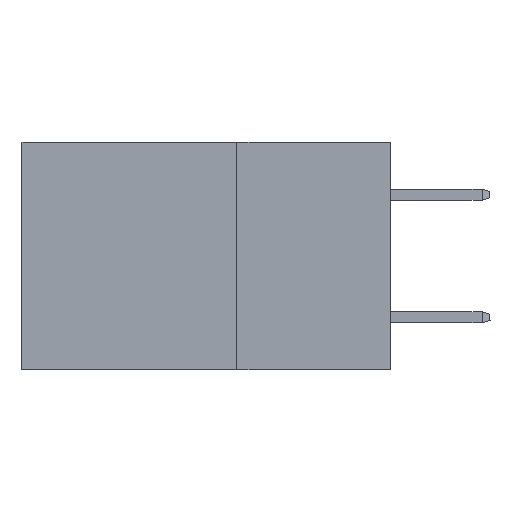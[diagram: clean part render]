
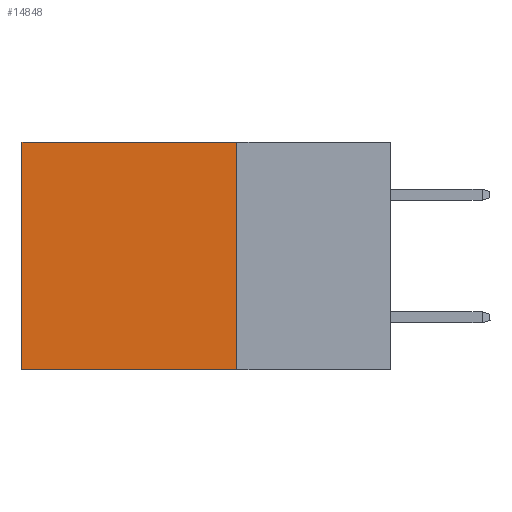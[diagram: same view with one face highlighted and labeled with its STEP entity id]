
A CAD part, left-side view. The second image highlights one B-rep face of the part: STEP entity #14848.
In plain terms, the highlighted planar face has unit normal (-1, 0, 0).
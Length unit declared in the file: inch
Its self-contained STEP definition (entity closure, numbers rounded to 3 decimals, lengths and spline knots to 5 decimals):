
#57 = EDGE_CURVE ( 'NONE', #25515, #14974, #1301, .T. ) ;
#1301 = LINE ( 'NONE', #20727, #3174 ) ;
#2214 = LINE ( 'NONE', #20636, #16234 ) ;
#3174 = VECTOR ( 'NONE', #24867, 39.37008 ) ;
#4526 = VECTOR ( 'NONE', #22218, 39.37008 ) ;
#6023 = CARTESIAN_POINT ( 'NONE',  ( 0.2875, 0.25, -0.37 ) ) ;
#7574 = EDGE_LOOP ( 'NONE', ( #11862, #17883, #24803, #11158 ) ) ;
#7950 = LINE ( 'NONE', #10287, #4526 ) ;
#8965 = PLANE ( 'NONE',  #15084 ) ;
#9404 = VECTOR ( 'NONE', #16774, 39.37008 ) ;
#10287 = CARTESIAN_POINT ( 'NONE',  ( 0.2875, 0.25, -0.37 ) ) ;
#10639 = DIRECTION ( 'NONE',  ( 0., 0., -1. ) ) ;
#11158 = ORIENTED_EDGE ( 'NONE', *, *, #15975, .T. ) ;
#11862 = ORIENTED_EDGE ( 'NONE', *, *, #57, .T. ) ;
#12198 = VERTEX_POINT ( 'NONE', #22595 ) ;
#14715 = LINE ( 'NONE', #20918, #9404 ) ;
#14848 = ADVANCED_FACE ( 'NONE', ( #20401 ), #8965, .F. ) ;
#14974 = VERTEX_POINT ( 'NONE', #17352 ) ;
#15084 = AXIS2_PLACEMENT_3D ( 'NONE', #18603, #22837, #10639 ) ;
#15472 = EDGE_CURVE ( 'NONE', #12198, #21016, #14715, .T. ) ;
#15975 = EDGE_CURVE ( 'NONE', #12198, #25515, #2214, .T. ) ;
#16234 = VECTOR ( 'NONE', #24873, 39.37008 ) ;
#16774 = DIRECTION ( 'NONE',  ( 0., 0., -1. ) ) ;
#17352 = CARTESIAN_POINT ( 'NONE',  ( 0.2875, 0.6, -0.37 ) ) ;
#17883 = ORIENTED_EDGE ( 'NONE', *, *, #23060, .F. ) ;
#18603 = CARTESIAN_POINT ( 'NONE',  ( 0.2875, 0.25, 0. ) ) ;
#20401 = FACE_OUTER_BOUND ( 'NONE', #7574, .T. ) ;
#20636 = CARTESIAN_POINT ( 'NONE',  ( 0.2875, 0.25, 0. ) ) ;
#20727 = CARTESIAN_POINT ( 'NONE',  ( 0.2875, 0.6, 0. ) ) ;
#20918 = CARTESIAN_POINT ( 'NONE',  ( 0.2875, 0.25, 0. ) ) ;
#21016 = VERTEX_POINT ( 'NONE', #6023 ) ;
#21943 = CARTESIAN_POINT ( 'NONE',  ( 0.2875, 0.6, 0. ) ) ;
#22218 = DIRECTION ( 'NONE',  ( 0., 1., 0. ) ) ;
#22595 = CARTESIAN_POINT ( 'NONE',  ( 0.2875, 0.25, 0. ) ) ;
#22837 = DIRECTION ( 'NONE',  ( 1., 0., 0. ) ) ;
#23060 = EDGE_CURVE ( 'NONE', #21016, #14974, #7950, .T. ) ;
#24803 = ORIENTED_EDGE ( 'NONE', *, *, #15472, .F. ) ;
#24867 = DIRECTION ( 'NONE',  ( 0., 0., -1. ) ) ;
#24873 = DIRECTION ( 'NONE',  ( 0., 1., 0. ) ) ;
#25515 = VERTEX_POINT ( 'NONE', #21943 ) ;
